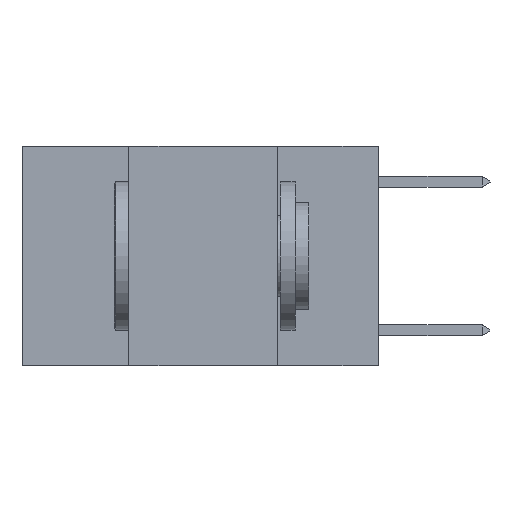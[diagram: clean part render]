
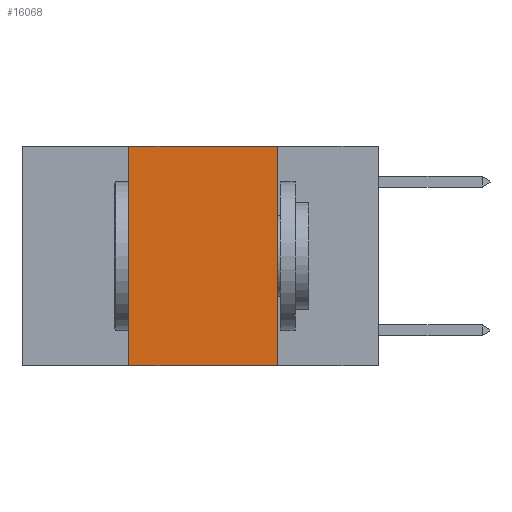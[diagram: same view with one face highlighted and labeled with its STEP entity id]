
A CAD part, left-side view. The second image highlights one B-rep face of the part: STEP entity #16068.
In plain terms, the highlighted planar face has unit normal (-1, 0, 0).
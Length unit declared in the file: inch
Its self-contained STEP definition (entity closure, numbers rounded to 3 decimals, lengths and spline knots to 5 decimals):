
#1955 = VECTOR ( 'NONE', #17286, 39.37008 ) ;
#2310 = CARTESIAN_POINT ( 'NONE',  ( 0., 0.42, 0. ) ) ;
#2854 = ORIENTED_EDGE ( 'NONE', *, *, #15147, .F. ) ;
#3366 = AXIS2_PLACEMENT_3D ( 'NONE', #26422, #13897, #31375 ) ;
#3819 = VERTEX_POINT ( 'NONE', #26607 ) ;
#6157 = VERTEX_POINT ( 'NONE', #25634 ) ;
#6562 = VECTOR ( 'NONE', #22968, 39.37008 ) ;
#8539 = VERTEX_POINT ( 'NONE', #11814 ) ;
#10005 = CARTESIAN_POINT ( 'NONE',  ( 0., 0.6, -0.37 ) ) ;
#10359 = CARTESIAN_POINT ( 'NONE',  ( 0., 0.17, 0. ) ) ;
#10798 = CARTESIAN_POINT ( 'NONE',  ( 0., 0.42, -0.37 ) ) ;
#11814 = CARTESIAN_POINT ( 'NONE',  ( 0., 0.17, -0.37 ) ) ;
#12392 = VECTOR ( 'NONE', #27634, 39.37008 ) ;
#13897 = DIRECTION ( 'NONE',  ( 1., 0., 0. ) ) ;
#14377 = ORIENTED_EDGE ( 'NONE', *, *, #17660, .F. ) ;
#14919 = DIRECTION ( 'NONE',  ( 0., 0., 1. ) ) ;
#15147 = EDGE_CURVE ( 'NONE', #3819, #8539, #20062, .T. ) ;
#15600 = LINE ( 'NONE', #10005, #12392 ) ;
#16068 = ADVANCED_FACE ( 'NONE', ( #31461 ), #28915, .F. ) ;
#16880 = EDGE_CURVE ( 'NONE', #6157, #3819, #27156, .T. ) ;
#17286 = DIRECTION ( 'NONE',  ( 0., -1., 0. ) ) ;
#17491 = ORIENTED_EDGE ( 'NONE', *, *, #16880, .F. ) ;
#17660 = EDGE_CURVE ( 'NONE', #23494, #6157, #25988, .T. ) ;
#20042 = VECTOR ( 'NONE', #14919, 39.37008 ) ;
#20062 = LINE ( 'NONE', #10359, #6562 ) ;
#22968 = DIRECTION ( 'NONE',  ( 0., 0., -1. ) ) ;
#23494 = VERTEX_POINT ( 'NONE', #10798 ) ;
#24262 = EDGE_LOOP ( 'NONE', ( #2854, #17491, #14377, #30032 ) ) ;
#25634 = CARTESIAN_POINT ( 'NONE',  ( 0., 0.42, 0. ) ) ;
#25988 = LINE ( 'NONE', #2310, #20042 ) ;
#26422 = CARTESIAN_POINT ( 'NONE',  ( 0., 0.6, 0. ) ) ;
#26607 = CARTESIAN_POINT ( 'NONE',  ( 0., 0.17, 0. ) ) ;
#27156 = LINE ( 'NONE', #32191, #1955 ) ;
#27634 = DIRECTION ( 'NONE',  ( 0., -1., 0. ) ) ;
#27953 = EDGE_CURVE ( 'NONE', #23494, #8539, #15600, .T. ) ;
#28915 = PLANE ( 'NONE',  #3366 ) ;
#30032 = ORIENTED_EDGE ( 'NONE', *, *, #27953, .T. ) ;
#31375 = DIRECTION ( 'NONE',  ( 0., 0., -1. ) ) ;
#31461 = FACE_OUTER_BOUND ( 'NONE', #24262, .T. ) ;
#32191 = CARTESIAN_POINT ( 'NONE',  ( 0., 0.6, 0. ) ) ;
